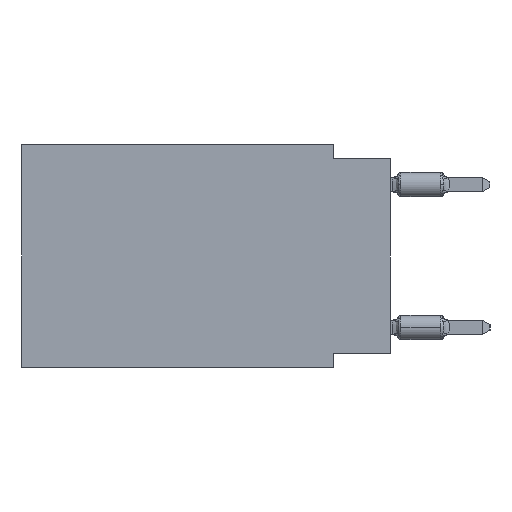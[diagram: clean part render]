
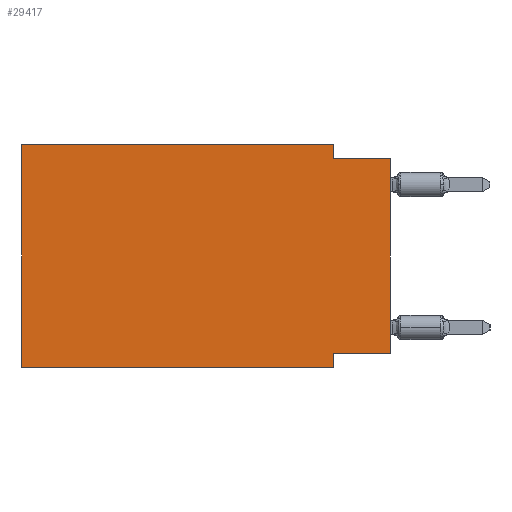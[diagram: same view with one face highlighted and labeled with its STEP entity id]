
A CAD part, left-side view. The second image highlights one B-rep face of the part: STEP entity #29417.
In plain terms, the highlighted planar face has unit normal (-1, 0, 0).
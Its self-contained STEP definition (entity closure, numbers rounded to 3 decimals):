
#347 = DIRECTION ( 'NONE',  ( 0., 0., 1. ) ) ;
#581 = DIRECTION ( 'NONE',  ( 0., 0., 1. ) ) ;
#813 = LINE ( 'NONE', #38242, #19637 ) ;
#1809 = DIRECTION ( 'NONE',  ( 1., 0., 0. ) ) ;
#1829 = AXIS2_PLACEMENT_3D ( 'NONE', #17815, #1809, #22700 ) ;
#3680 = CARTESIAN_POINT ( 'NONE',  ( 0., 2.54, -9.906 ) ) ;
#3892 = LINE ( 'NONE', #36975, #25953 ) ;
#6145 = FACE_OUTER_BOUND ( 'NONE', #45892, .T. ) ;
#6445 = ORIENTED_EDGE ( 'NONE', *, *, #22916, .T. ) ;
#7175 = ORIENTED_EDGE ( 'NONE', *, *, #43827, .F. ) ;
#8027 = ORIENTED_EDGE ( 'NONE', *, *, #33269, .F. ) ;
#8892 = CARTESIAN_POINT ( 'NONE',  ( 0., 2.54, -9.906 ) ) ;
#10399 = CARTESIAN_POINT ( 'NONE',  ( 0., 0., -0.635 ) ) ;
#10500 = VECTOR ( 'NONE', #12613, 1000. ) ;
#12520 = CARTESIAN_POINT ( 'NONE',  ( 0., 0., 0. ) ) ;
#12613 = DIRECTION ( 'NONE',  ( 0., 1., 0. ) ) ;
#12901 = VERTEX_POINT ( 'NONE', #15149 ) ;
#13335 = VERTEX_POINT ( 'NONE', #22965 ) ;
#14383 = CARTESIAN_POINT ( 'NONE',  ( 0., 16.383, -9.906 ) ) ;
#14971 = CARTESIAN_POINT ( 'NONE',  ( 0., 2.54, -0.635 ) ) ;
#15149 = CARTESIAN_POINT ( 'NONE',  ( 0., 2.54, -9.271 ) ) ;
#15885 = EDGE_CURVE ( 'NONE', #30483, #12901, #24563, .T. ) ;
#16745 = ORIENTED_EDGE ( 'NONE', *, *, #33613, .T. ) ;
#17372 = DIRECTION ( 'NONE',  ( 0., -1., 0. ) ) ;
#17815 = CARTESIAN_POINT ( 'NONE',  ( 0., 16.383, 0. ) ) ;
#19041 = VERTEX_POINT ( 'NONE', #14971 ) ;
#19404 = ORIENTED_EDGE ( 'NONE', *, *, #50777, .F. ) ;
#19637 = VECTOR ( 'NONE', #17372, 1000. ) ;
#20896 = CARTESIAN_POINT ( 'NONE',  ( 0., 0., -9.271 ) ) ;
#21454 = ORIENTED_EDGE ( 'NONE', *, *, #49039, .F. ) ;
#22700 = DIRECTION ( 'NONE',  ( 0., 0., -1. ) ) ;
#22916 = EDGE_CURVE ( 'NONE', #40357, #38695, #813, .T. ) ;
#22965 = CARTESIAN_POINT ( 'NONE',  ( 0., 0., -0.635 ) ) ;
#24190 = LINE ( 'NONE', #36643, #47463 ) ;
#24563 = LINE ( 'NONE', #37024, #10500 ) ;
#25953 = VECTOR ( 'NONE', #53510, 1000. ) ;
#26141 = CARTESIAN_POINT ( 'NONE',  ( 0., 16.383, 0. ) ) ;
#28911 = DIRECTION ( 'NONE',  ( 0., 0., -1. ) ) ;
#28973 = CARTESIAN_POINT ( 'NONE',  ( 0., 2.54, 0. ) ) ;
#29417 = ADVANCED_FACE ( 'NONE', ( #6145 ), #31389, .F. ) ;
#29942 = VERTEX_POINT ( 'NONE', #48879 ) ;
#30483 = VERTEX_POINT ( 'NONE', #20896 ) ;
#31389 = PLANE ( 'NONE',  #1829 ) ;
#32405 = VECTOR ( 'NONE', #51606, 1000. ) ;
#33269 = EDGE_CURVE ( 'NONE', #19041, #13335, #46994, .T. ) ;
#33417 = LINE ( 'NONE', #12520, #48026 ) ;
#33613 = EDGE_CURVE ( 'NONE', #30483, #13335, #33417, .T. ) ;
#34303 = ORIENTED_EDGE ( 'NONE', *, *, #50903, .F. ) ;
#35493 = VECTOR ( 'NONE', #347, 1000. ) ;
#36643 = CARTESIAN_POINT ( 'NONE',  ( 0., 16.383, 0. ) ) ;
#36975 = CARTESIAN_POINT ( 'NONE',  ( 0., 2.54, 0. ) ) ;
#37024 = CARTESIAN_POINT ( 'NONE',  ( 0., 0., -9.271 ) ) ;
#38049 = LINE ( 'NONE', #26141, #35493 ) ;
#38242 = CARTESIAN_POINT ( 'NONE',  ( 0., 16.383, -9.906 ) ) ;
#38695 = VERTEX_POINT ( 'NONE', #8892 ) ;
#38722 = VERTEX_POINT ( 'NONE', #28973 ) ;
#39835 = ORIENTED_EDGE ( 'NONE', *, *, #15885, .F. ) ;
#40357 = VERTEX_POINT ( 'NONE', #14383 ) ;
#40833 = LINE ( 'NONE', #3680, #52787 ) ;
#43827 = EDGE_CURVE ( 'NONE', #29942, #38722, #24190, .T. ) ;
#44778 = DIRECTION ( 'NONE',  ( 0., -1., 0. ) ) ;
#45892 = EDGE_LOOP ( 'NONE', ( #16745, #8027, #19404, #7175, #34303, #6445, #21454, #39835 ) ) ;
#46994 = LINE ( 'NONE', #10399, #32405 ) ;
#47463 = VECTOR ( 'NONE', #44778, 1000. ) ;
#48026 = VECTOR ( 'NONE', #581, 1000. ) ;
#48879 = CARTESIAN_POINT ( 'NONE',  ( 0., 16.383, 0. ) ) ;
#49039 = EDGE_CURVE ( 'NONE', #12901, #38695, #40833, .T. ) ;
#50777 = EDGE_CURVE ( 'NONE', #38722, #19041, #3892, .T. ) ;
#50903 = EDGE_CURVE ( 'NONE', #40357, #29942, #38049, .T. ) ;
#51606 = DIRECTION ( 'NONE',  ( 0., -1., 0. ) ) ;
#52787 = VECTOR ( 'NONE', #28911, 1000. ) ;
#53510 = DIRECTION ( 'NONE',  ( 0., 0., -1. ) ) ;
